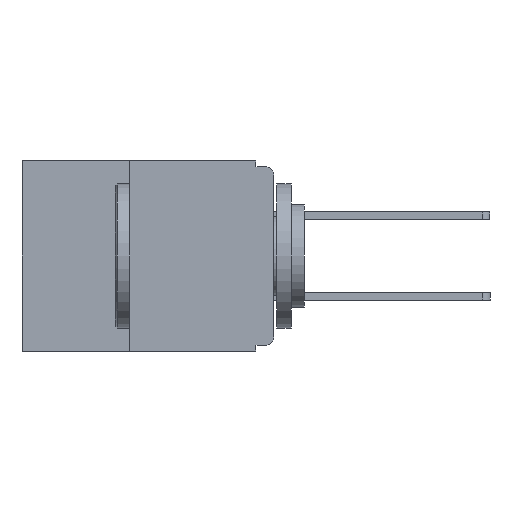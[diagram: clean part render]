
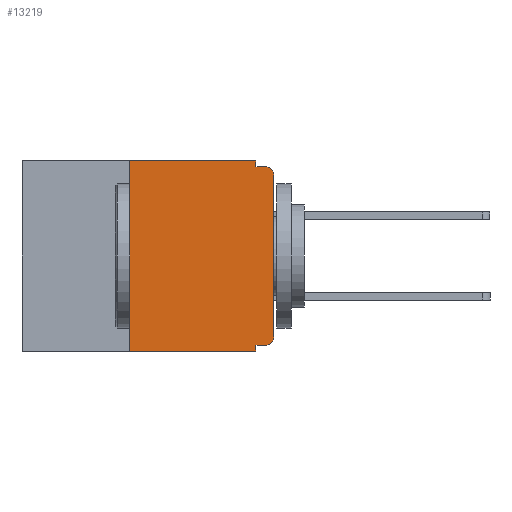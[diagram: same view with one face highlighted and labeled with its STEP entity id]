
A CAD part, left-side view. The second image highlights one B-rep face of the part: STEP entity #13219.
In plain terms, the highlighted planar face has unit normal (-1, 0, 0).
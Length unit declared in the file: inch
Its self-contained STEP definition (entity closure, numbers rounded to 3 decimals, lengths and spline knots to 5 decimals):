
#223 = LINE ( 'NONE', #24332, #34134 ) ;
#704 = ORIENTED_EDGE ( 'NONE', *, *, #24131, .F. ) ;
#1357 = VERTEX_POINT ( 'NONE', #26440 ) ;
#1367 = LINE ( 'NONE', #4225, #14977 ) ;
#1405 = ORIENTED_EDGE ( 'NONE', *, *, #7503, .F. ) ;
#2233 = LINE ( 'NONE', #33694, #23721 ) ;
#4225 = CARTESIAN_POINT ( 'NONE',  ( 0., 0., -0.32 ) ) ;
#5415 = CARTESIAN_POINT ( 'NONE',  ( 0., 0.437, -0.33 ) ) ;
#5472 = VERTEX_POINT ( 'NONE', #14948 ) ;
#6218 = AXIS2_PLACEMENT_3D ( 'NONE', #6553, #25258, #9286 ) ;
#6553 = CARTESIAN_POINT ( 'NONE',  ( 0., 0.437, 0. ) ) ;
#6612 = EDGE_CURVE ( 'NONE', #1357, #24423, #24113, .T. ) ;
#7012 = DIRECTION ( 'NONE',  ( 0., 1., 0. ) ) ;
#7503 = EDGE_CURVE ( 'NONE', #7508, #22913, #21167, .T. ) ;
#7508 = VERTEX_POINT ( 'NONE', #21999 ) ;
#7973 = CARTESIAN_POINT ( 'NONE',  ( 0., 0.25, 0. ) ) ;
#8902 = VECTOR ( 'NONE', #17386, 39.37008 ) ;
#9286 = DIRECTION ( 'NONE',  ( 0., 0., -1. ) ) ;
#9747 = LINE ( 'NONE', #33239, #8902 ) ;
#9812 = CARTESIAN_POINT ( 'NONE',  ( 0., 0.031, -0.33 ) ) ;
#9872 = EDGE_CURVE ( 'NONE', #24423, #17343, #31719, .T. ) ;
#10164 = VERTEX_POINT ( 'NONE', #7973 ) ;
#10537 = VECTOR ( 'NONE', #12941, 39.37008 ) ;
#11471 = LINE ( 'NONE', #24402, #34642 ) ;
#11957 = DIRECTION ( 'NONE',  ( 0., 0., -1. ) ) ;
#11966 = DIRECTION ( 'NONE',  ( -1., 0., 0. ) ) ;
#11993 = CARTESIAN_POINT ( 'NONE',  ( 0., 0.015, -0.305 ) ) ;
#12161 = EDGE_CURVE ( 'NONE', #27890, #10164, #2233, .T. ) ;
#12534 = AXIS2_PLACEMENT_3D ( 'NONE', #11993, #11966, #11957 ) ;
#12858 = CARTESIAN_POINT ( 'NONE',  ( 0., 0., 0. ) ) ;
#12941 = DIRECTION ( 'NONE',  ( 0., 0., 1. ) ) ;
#13219 = ADVANCED_FACE ( 'NONE', ( #31538 ), #30441, .F. ) ;
#13451 = CIRCLE ( 'NONE', #17937, 0.015 ) ;
#14663 = DIRECTION ( 'NONE',  ( -1., 0., 0. ) ) ;
#14883 = CARTESIAN_POINT ( 'NONE',  ( 0., 0., -0.305 ) ) ;
#14948 = CARTESIAN_POINT ( 'NONE',  ( 0., 0.031, 0. ) ) ;
#14977 = VECTOR ( 'NONE', #7012, 39.37008 ) ;
#16289 = DIRECTION ( 'NONE',  ( 0., 0., -1. ) ) ;
#16471 = DIRECTION ( 'NONE',  ( 0., -1., 0. ) ) ;
#16906 = ORIENTED_EDGE ( 'NONE', *, *, #24366, .T. ) ;
#17343 = VERTEX_POINT ( 'NONE', #32215 ) ;
#17386 = DIRECTION ( 'NONE',  ( 0., -1., 0. ) ) ;
#17692 = ORIENTED_EDGE ( 'NONE', *, *, #30386, .F. ) ;
#17937 = AXIS2_PLACEMENT_3D ( 'NONE', #30537, #14663, #33161 ) ;
#19633 = ORIENTED_EDGE ( 'NONE', *, *, #22619, .F. ) ;
#20288 = ORIENTED_EDGE ( 'NONE', *, *, #27741, .F. ) ;
#20813 = VERTEX_POINT ( 'NONE', #32284 ) ;
#21167 = LINE ( 'NONE', #22160, #28191 ) ;
#21999 = CARTESIAN_POINT ( 'NONE',  ( 0., 0.031, -0.32 ) ) ;
#22160 = CARTESIAN_POINT ( 'NONE',  ( 0., 0.031, -0.33 ) ) ;
#22416 = DIRECTION ( 'NONE',  ( 0., 0., -1. ) ) ;
#22619 = EDGE_CURVE ( 'NONE', #25113, #20813, #11471, .T. ) ;
#22913 = VERTEX_POINT ( 'NONE', #9812 ) ;
#23117 = DIRECTION ( 'NONE',  ( 0., 0., 1. ) ) ;
#23721 = VECTOR ( 'NONE', #23117, 39.37008 ) ;
#23840 = EDGE_LOOP ( 'NONE', ( #29136, #16906, #19633, #704, #20288, #30239, #32725, #1405, #17692, #26099 ) ) ;
#24113 = CIRCLE ( 'NONE', #12534, 0.015 ) ;
#24131 = EDGE_CURVE ( 'NONE', #5472, #25113, #223, .T. ) ;
#24332 = CARTESIAN_POINT ( 'NONE',  ( 0., 0.031, 0. ) ) ;
#24366 = EDGE_CURVE ( 'NONE', #17343, #20813, #13451, .T. ) ;
#24402 = CARTESIAN_POINT ( 'NONE',  ( 0., 0., -0.01 ) ) ;
#24423 = VERTEX_POINT ( 'NONE', #14883 ) ;
#25113 = VERTEX_POINT ( 'NONE', #31074 ) ;
#25258 = DIRECTION ( 'NONE',  ( 1., 0., 0. ) ) ;
#26099 = ORIENTED_EDGE ( 'NONE', *, *, #6612, .T. ) ;
#26440 = CARTESIAN_POINT ( 'NONE',  ( 0., 0.015, -0.32 ) ) ;
#26845 = DIRECTION ( 'NONE',  ( 0., -1., 0. ) ) ;
#27016 = VECTOR ( 'NONE', #26845, 39.37008 ) ;
#27741 = EDGE_CURVE ( 'NONE', #10164, #5472, #9747, .T. ) ;
#27846 = LINE ( 'NONE', #5415, #27016 ) ;
#27890 = VERTEX_POINT ( 'NONE', #28626 ) ;
#28191 = VECTOR ( 'NONE', #22416, 39.37008 ) ;
#28626 = CARTESIAN_POINT ( 'NONE',  ( 0., 0.25, -0.33 ) ) ;
#29136 = ORIENTED_EDGE ( 'NONE', *, *, #9872, .T. ) ;
#30239 = ORIENTED_EDGE ( 'NONE', *, *, #12161, .F. ) ;
#30386 = EDGE_CURVE ( 'NONE', #1357, #7508, #1367, .T. ) ;
#30441 = PLANE ( 'NONE',  #6218 ) ;
#30537 = CARTESIAN_POINT ( 'NONE',  ( 0., 0.015, -0.025 ) ) ;
#30650 = EDGE_CURVE ( 'NONE', #27890, #22913, #27846, .T. ) ;
#31074 = CARTESIAN_POINT ( 'NONE',  ( 0., 0.031, -0.01 ) ) ;
#31538 = FACE_OUTER_BOUND ( 'NONE', #23840, .T. ) ;
#31719 = LINE ( 'NONE', #12858, #10537 ) ;
#32215 = CARTESIAN_POINT ( 'NONE',  ( 0., 0., -0.025 ) ) ;
#32284 = CARTESIAN_POINT ( 'NONE',  ( 0., 0.015, -0.01 ) ) ;
#32725 = ORIENTED_EDGE ( 'NONE', *, *, #30650, .T. ) ;
#33161 = DIRECTION ( 'NONE',  ( 0., 0., -1. ) ) ;
#33239 = CARTESIAN_POINT ( 'NONE',  ( 0., 0.437, 0. ) ) ;
#33694 = CARTESIAN_POINT ( 'NONE',  ( 0., 0.25, -0.33 ) ) ;
#34134 = VECTOR ( 'NONE', #16289, 39.37008 ) ;
#34642 = VECTOR ( 'NONE', #16471, 39.37008 ) ;
